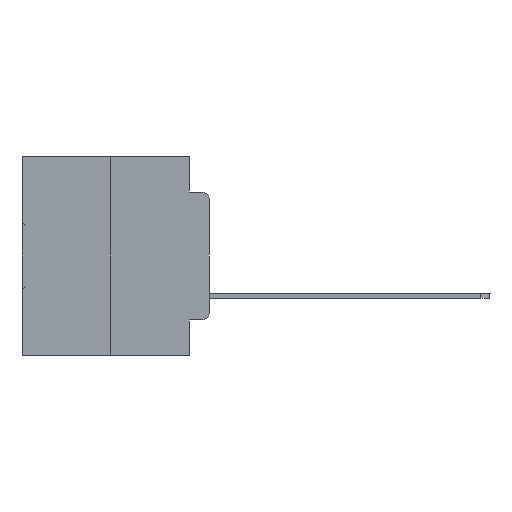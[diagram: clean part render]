
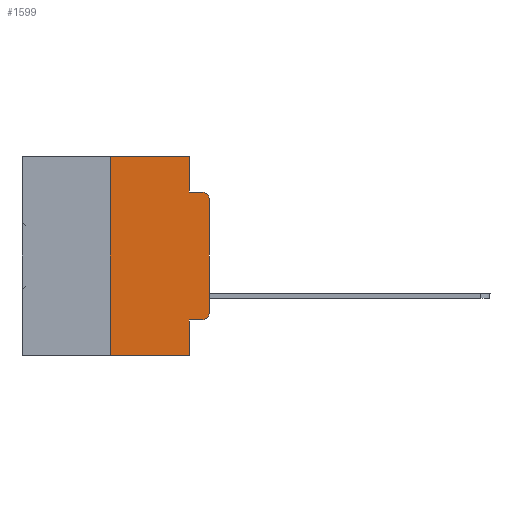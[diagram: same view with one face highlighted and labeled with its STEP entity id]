
A CAD part, left-side view. The second image highlights one B-rep face of the part: STEP entity #1599.
In plain terms, the highlighted planar face has unit normal (-1, 0, 0).
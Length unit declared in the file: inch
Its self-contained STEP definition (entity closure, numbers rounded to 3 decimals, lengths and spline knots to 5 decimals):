
#151 = CIRCLE ( 'NONE', #34095, 0.02 ) ;
#404 = DIRECTION ( 'NONE',  ( 0., -1., 0. ) ) ;
#530 = DIRECTION ( 'NONE',  ( 0., 0., -1. ) ) ;
#729 = EDGE_CURVE ( 'NONE', #1594, #14573, #8581, .T. ) ;
#762 = PLANE ( 'NONE',  #29518 ) ;
#1063 = ORIENTED_EDGE ( 'NONE', *, *, #2383, .F. ) ;
#1150 = ORIENTED_EDGE ( 'NONE', *, *, #15770, .T. ) ;
#1594 = VERTEX_POINT ( 'NONE', #30768 ) ;
#1599 = ADVANCED_FACE ( 'NONE', ( #11599 ), #762, .F. ) ;
#1836 = CARTESIAN_POINT ( 'NONE',  ( 0., 0., -0.1085 ) ) ;
#2383 = EDGE_CURVE ( 'NONE', #4761, #12451, #10299, .T. ) ;
#2569 = DIRECTION ( 'NONE',  ( -1., 0., 0. ) ) ;
#3029 = CARTESIAN_POINT ( 'NONE',  ( 0., 0.02, -0.1085 ) ) ;
#3231 = EDGE_LOOP ( 'NONE', ( #4311, #1150, #15484, #1063, #17163, #34299, #18778, #28573, #26079, #27155 ) ) ;
#4311 = ORIENTED_EDGE ( 'NONE', *, *, #9414, .T. ) ;
#4343 = CARTESIAN_POINT ( 'NONE',  ( 0., 0.473, 0. ) ) ;
#4681 = LINE ( 'NONE', #4343, #19751 ) ;
#4761 = VERTEX_POINT ( 'NONE', #12265 ) ;
#5771 = CARTESIAN_POINT ( 'NONE',  ( 0., 0.051, -0.0885 ) ) ;
#5931 = EDGE_CURVE ( 'NONE', #11485, #14573, #34333, .T. ) ;
#6000 = CARTESIAN_POINT ( 'NONE',  ( 0., 0.051, -0.5 ) ) ;
#6155 = DIRECTION ( 'NONE',  ( 0., 0., 1. ) ) ;
#7129 = EDGE_CURVE ( 'NONE', #26191, #25101, #151, .T. ) ;
#7412 = CARTESIAN_POINT ( 'NONE',  ( 0., 0.02, -0.0885 ) ) ;
#8150 = AXIS2_PLACEMENT_3D ( 'NONE', #3029, #16131, #26607 ) ;
#8581 = LINE ( 'NONE', #16768, #26418 ) ;
#9414 = EDGE_CURVE ( 'NONE', #25101, #12852, #14023, .T. ) ;
#9929 = CARTESIAN_POINT ( 'NONE',  ( 0., 0.051, -0.0885 ) ) ;
#10299 = LINE ( 'NONE', #26354, #25714 ) ;
#11369 = DIRECTION ( 'NONE',  ( 0., -1., 0. ) ) ;
#11485 = VERTEX_POINT ( 'NONE', #22905 ) ;
#11599 = FACE_OUTER_BOUND ( 'NONE', #3231, .T. ) ;
#12053 = CIRCLE ( 'NONE', #8150, 0.02 ) ;
#12265 = CARTESIAN_POINT ( 'NONE',  ( 0., 0.051, 0. ) ) ;
#12367 = DIRECTION ( 'NONE',  ( 0., -1., 0. ) ) ;
#12451 = VERTEX_POINT ( 'NONE', #9929 ) ;
#12852 = VERTEX_POINT ( 'NONE', #1836 ) ;
#13049 = VECTOR ( 'NONE', #6155, 39.37008 ) ;
#13090 = DIRECTION ( 'NONE',  ( 0., 0., -1. ) ) ;
#13498 = CARTESIAN_POINT ( 'NONE',  ( 0., 0., 0. ) ) ;
#14023 = LINE ( 'NONE', #13498, #13049 ) ;
#14129 = VECTOR ( 'NONE', #11369, 39.37008 ) ;
#14386 = DIRECTION ( 'NONE',  ( 1., 0., 0. ) ) ;
#14573 = VERTEX_POINT ( 'NONE', #6000 ) ;
#15484 = ORIENTED_EDGE ( 'NONE', *, *, #29074, .F. ) ;
#15507 = CARTESIAN_POINT ( 'NONE',  ( 0., 0.02, -0.3915 ) ) ;
#15745 = CARTESIAN_POINT ( 'NONE',  ( 0., 0., -0.3915 ) ) ;
#15770 = EDGE_CURVE ( 'NONE', #12852, #21394, #12053, .T. ) ;
#15788 = EDGE_CURVE ( 'NONE', #1594, #26191, #16655, .T. ) ;
#16131 = DIRECTION ( 'NONE',  ( -1., 0., 0. ) ) ;
#16360 = CARTESIAN_POINT ( 'NONE',  ( 0., 0.473, -0.5 ) ) ;
#16655 = LINE ( 'NONE', #27300, #25987 ) ;
#16768 = CARTESIAN_POINT ( 'NONE',  ( 0., 0.051, 0. ) ) ;
#16981 = VECTOR ( 'NONE', #17947, 39.37008 ) ;
#17163 = ORIENTED_EDGE ( 'NONE', *, *, #32049, .F. ) ;
#17431 = CARTESIAN_POINT ( 'NONE',  ( 0., 0.25, 0. ) ) ;
#17505 = DIRECTION ( 'NONE',  ( 0., 0., -1. ) ) ;
#17947 = DIRECTION ( 'NONE',  ( 0., 0., 1. ) ) ;
#18778 = ORIENTED_EDGE ( 'NONE', *, *, #5931, .T. ) ;
#19751 = VECTOR ( 'NONE', #12367, 39.37008 ) ;
#21394 = VERTEX_POINT ( 'NONE', #7412 ) ;
#22823 = LINE ( 'NONE', #17431, #16981 ) ;
#22905 = CARTESIAN_POINT ( 'NONE',  ( 0., 0.25, -0.5 ) ) ;
#24645 = VECTOR ( 'NONE', #31708, 39.37008 ) ;
#25101 = VERTEX_POINT ( 'NONE', #15745 ) ;
#25714 = VECTOR ( 'NONE', #13090, 39.37008 ) ;
#25987 = VECTOR ( 'NONE', #404, 39.37008 ) ;
#26079 = ORIENTED_EDGE ( 'NONE', *, *, #15788, .T. ) ;
#26191 = VERTEX_POINT ( 'NONE', #32754 ) ;
#26354 = CARTESIAN_POINT ( 'NONE',  ( 0., 0.051, 0. ) ) ;
#26418 = VECTOR ( 'NONE', #530, 39.37008 ) ;
#26607 = DIRECTION ( 'NONE',  ( 0., 0., -1. ) ) ;
#27155 = ORIENTED_EDGE ( 'NONE', *, *, #7129, .T. ) ;
#27300 = CARTESIAN_POINT ( 'NONE',  ( 0., 0.051, -0.4115 ) ) ;
#28573 = ORIENTED_EDGE ( 'NONE', *, *, #729, .F. ) ;
#28854 = VERTEX_POINT ( 'NONE', #32510 ) ;
#29074 = EDGE_CURVE ( 'NONE', #12451, #21394, #29680, .T. ) ;
#29518 = AXIS2_PLACEMENT_3D ( 'NONE', #30260, #14386, #17505 ) ;
#29680 = LINE ( 'NONE', #5771, #14129 ) ;
#30260 = CARTESIAN_POINT ( 'NONE',  ( 0., 0.473, 0. ) ) ;
#30768 = CARTESIAN_POINT ( 'NONE',  ( 0., 0.051, -0.4115 ) ) ;
#31549 = DIRECTION ( 'NONE',  ( 0., 0., -1. ) ) ;
#31708 = DIRECTION ( 'NONE',  ( 0., -1., 0. ) ) ;
#32049 = EDGE_CURVE ( 'NONE', #28854, #4761, #4681, .T. ) ;
#32083 = EDGE_CURVE ( 'NONE', #11485, #28854, #22823, .T. ) ;
#32510 = CARTESIAN_POINT ( 'NONE',  ( 0., 0.25, 0. ) ) ;
#32754 = CARTESIAN_POINT ( 'NONE',  ( 0., 0.02, -0.4115 ) ) ;
#34095 = AXIS2_PLACEMENT_3D ( 'NONE', #15507, #2569, #31549 ) ;
#34299 = ORIENTED_EDGE ( 'NONE', *, *, #32083, .F. ) ;
#34333 = LINE ( 'NONE', #16360, #24645 ) ;
